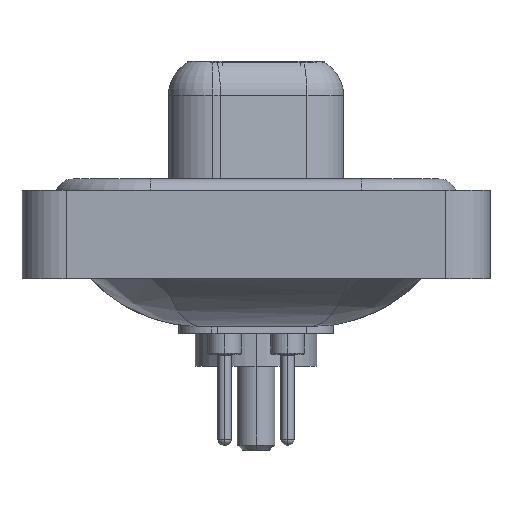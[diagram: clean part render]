
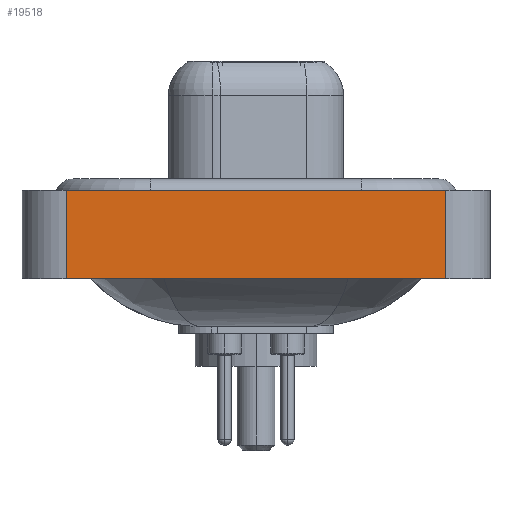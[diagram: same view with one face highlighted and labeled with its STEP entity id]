
A CAD part, left-side view. The second image highlights one B-rep face of the part: STEP entity #19518.
In plain terms, the highlighted planar face has unit normal (-1, 0, 0).
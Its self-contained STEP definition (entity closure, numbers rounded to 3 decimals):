
#144 = VERTEX_POINT ( 'NONE', #5824 ) ;
#1022 = DIRECTION ( 'NONE',  ( 0., -1., 0. ) ) ;
#1522 = LINE ( 'NONE', #13381, #5677 ) ;
#1531 = EDGE_CURVE ( 'NONE', #9037, #144, #13337, .T. ) ;
#1748 = EDGE_CURVE ( 'NONE', #6460, #2912, #2841, .T. ) ;
#1909 = VECTOR ( 'NONE', #3119, 1000. ) ;
#2244 = DIRECTION ( 'NONE',  ( -1., 0., 0. ) ) ;
#2250 = EDGE_CURVE ( 'NONE', #6460, #9037, #7034, .T. ) ;
#2841 = LINE ( 'NONE', #15094, #1909 ) ;
#2912 = VERTEX_POINT ( 'NONE', #14005 ) ;
#3119 = DIRECTION ( 'NONE',  ( 0., 0., 1. ) ) ;
#3179 = VECTOR ( 'NONE', #1022, 1000. ) ;
#3909 = ORIENTED_EDGE ( 'NONE', *, *, #1748, .F. ) ;
#4428 = DIRECTION ( 'NONE',  ( 0., -1., 0. ) ) ;
#5618 = CARTESIAN_POINT ( 'NONE',  ( -7.25, 8.55, -3.6 ) ) ;
#5677 = VECTOR ( 'NONE', #4428, 1000. ) ;
#5824 = CARTESIAN_POINT ( 'NONE',  ( -7.25, -8.55, 0.4 ) ) ;
#6194 = EDGE_CURVE ( 'NONE', #2912, #144, #1522, .T. ) ;
#6460 = VERTEX_POINT ( 'NONE', #5618 ) ;
#7034 = LINE ( 'NONE', #17911, #3179 ) ;
#9037 = VERTEX_POINT ( 'NONE', #17391 ) ;
#10270 = AXIS2_PLACEMENT_3D ( 'NONE', #15998, #2244, #17918 ) ;
#11764 = FACE_OUTER_BOUND ( 'NONE', #15344, .T. ) ;
#12642 = ORIENTED_EDGE ( 'NONE', *, *, #6194, .F. ) ;
#13337 = LINE ( 'NONE', #19088, #19873 ) ;
#13381 = CARTESIAN_POINT ( 'NONE',  ( -7.25, -8.55, 0.4 ) ) ;
#14005 = CARTESIAN_POINT ( 'NONE',  ( -7.25, 8.55, 0.4 ) ) ;
#15094 = CARTESIAN_POINT ( 'NONE',  ( -7.25, 8.55, -3.6 ) ) ;
#15344 = EDGE_LOOP ( 'NONE', ( #17830, #12642, #3909, #18546 ) ) ;
#15998 = CARTESIAN_POINT ( 'NONE',  ( -7.25, -8.55, -3.6 ) ) ;
#17391 = CARTESIAN_POINT ( 'NONE',  ( -7.25, -8.55, -3.6 ) ) ;
#17830 = ORIENTED_EDGE ( 'NONE', *, *, #1531, .T. ) ;
#17911 = CARTESIAN_POINT ( 'NONE',  ( -7.25, -8.55, -3.6 ) ) ;
#17918 = DIRECTION ( 'NONE',  ( 0., 0., 1. ) ) ;
#18546 = ORIENTED_EDGE ( 'NONE', *, *, #2250, .T. ) ;
#19088 = CARTESIAN_POINT ( 'NONE',  ( -7.25, -8.55, -3.6 ) ) ;
#19278 = DIRECTION ( 'NONE',  ( 0., 0., 1. ) ) ;
#19427 = PLANE ( 'NONE',  #10270 ) ;
#19518 = ADVANCED_FACE ( 'NONE', ( #11764 ), #19427, .T. ) ;
#19873 = VECTOR ( 'NONE', #19278, 1000. ) ;
